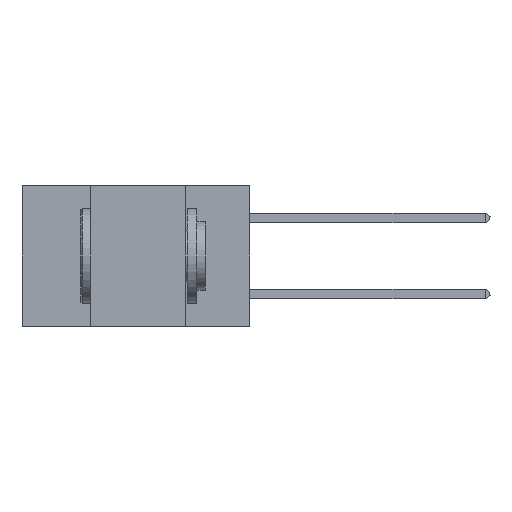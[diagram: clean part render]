
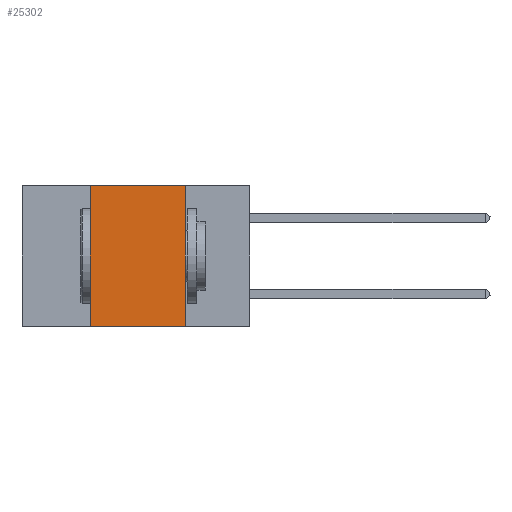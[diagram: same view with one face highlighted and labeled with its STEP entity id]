
A CAD part, left-side view. The second image highlights one B-rep face of the part: STEP entity #25302.
In plain terms, the highlighted planar face has unit normal (-1, 0, 0).
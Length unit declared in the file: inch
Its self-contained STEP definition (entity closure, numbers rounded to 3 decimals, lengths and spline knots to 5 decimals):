
#1784 = CARTESIAN_POINT ( 'NONE',  ( 0., 0.42, 0. ) ) ;
#2914 = DIRECTION ( 'NONE',  ( 0., -1., 0. ) ) ;
#3149 = CARTESIAN_POINT ( 'NONE',  ( 0., 0.6, 0. ) ) ;
#4556 = AXIS2_PLACEMENT_3D ( 'NONE', #3149, #40277, #6766 ) ;
#5448 = ORIENTED_EDGE ( 'NONE', *, *, #35892, .F. ) ;
#5694 = VERTEX_POINT ( 'NONE', #26669 ) ;
#6403 = FACE_OUTER_BOUND ( 'NONE', #25587, .T. ) ;
#6766 = DIRECTION ( 'NONE',  ( 0., 0., -1. ) ) ;
#10392 = CARTESIAN_POINT ( 'NONE',  ( 0., 0.6, -0.37 ) ) ;
#13832 = VERTEX_POINT ( 'NONE', #44071 ) ;
#20394 = LINE ( 'NONE', #39407, #47383 ) ;
#21967 = ORIENTED_EDGE ( 'NONE', *, *, #29389, .F. ) ;
#22098 = EDGE_CURVE ( 'NONE', #13832, #5694, #38844, .T. ) ;
#22624 = ORIENTED_EDGE ( 'NONE', *, *, #24088, .T. ) ;
#24088 = EDGE_CURVE ( 'NONE', #27164, #5694, #29455, .T. ) ;
#25302 = ADVANCED_FACE ( 'NONE', ( #6403 ), #32891, .F. ) ;
#25587 = EDGE_LOOP ( 'NONE', ( #31755, #21967, #5448, #22624 ) ) ;
#26669 = CARTESIAN_POINT ( 'NONE',  ( 0., 0.17, -0.37 ) ) ;
#27155 = VECTOR ( 'NONE', #47085, 39.37008 ) ;
#27164 = VERTEX_POINT ( 'NONE', #27582 ) ;
#27582 = CARTESIAN_POINT ( 'NONE',  ( 0., 0.42, -0.37 ) ) ;
#29389 = EDGE_CURVE ( 'NONE', #36645, #13832, #20394, .T. ) ;
#29455 = LINE ( 'NONE', #10392, #27155 ) ;
#31755 = ORIENTED_EDGE ( 'NONE', *, *, #22098, .F. ) ;
#31909 = DIRECTION ( 'NONE',  ( 0., 0., -1. ) ) ;
#32891 = PLANE ( 'NONE',  #4556 ) ;
#34625 = CARTESIAN_POINT ( 'NONE',  ( 0., 0.17, 0. ) ) ;
#34940 = DIRECTION ( 'NONE',  ( 0., 0., 1. ) ) ;
#35892 = EDGE_CURVE ( 'NONE', #27164, #36645, #46124, .T. ) ;
#36645 = VERTEX_POINT ( 'NONE', #39845 ) ;
#37160 = VECTOR ( 'NONE', #31909, 39.37008 ) ;
#38844 = LINE ( 'NONE', #34625, #37160 ) ;
#39407 = CARTESIAN_POINT ( 'NONE',  ( 0., 0.6, 0. ) ) ;
#39845 = CARTESIAN_POINT ( 'NONE',  ( 0., 0.42, 0. ) ) ;
#40277 = DIRECTION ( 'NONE',  ( 1., 0., 0. ) ) ;
#44071 = CARTESIAN_POINT ( 'NONE',  ( 0., 0.17, 0. ) ) ;
#46124 = LINE ( 'NONE', #1784, #46665 ) ;
#46665 = VECTOR ( 'NONE', #34940, 39.37008 ) ;
#47085 = DIRECTION ( 'NONE',  ( 0., -1., 0. ) ) ;
#47383 = VECTOR ( 'NONE', #2914, 39.37008 ) ;
